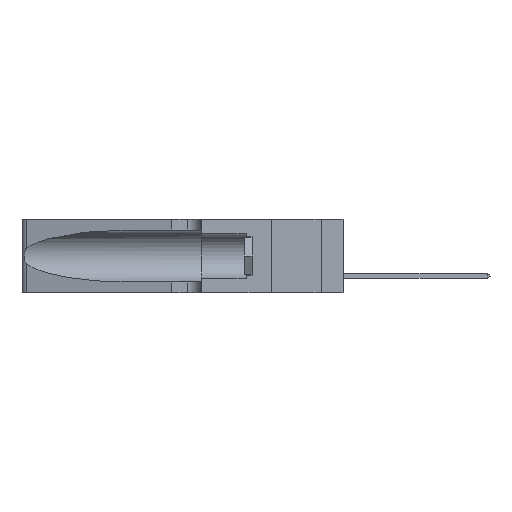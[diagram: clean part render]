
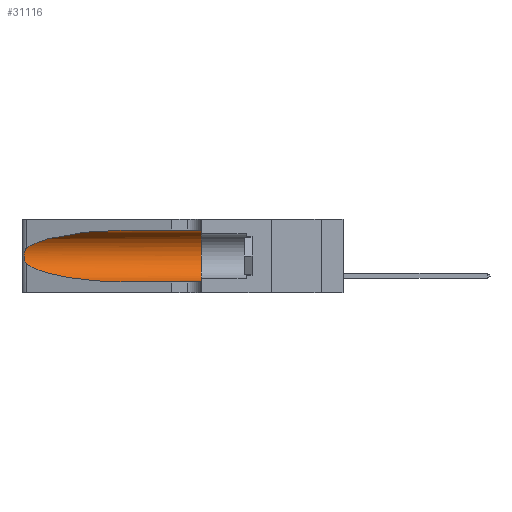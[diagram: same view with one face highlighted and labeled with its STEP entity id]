
A CAD part, left-side view. The second image highlights one B-rep face of the part: STEP entity #31116.
In plain terms, the highlighted cylindrical face has radius 3.308 mm (diameter 6.617 mm), a partial arc.
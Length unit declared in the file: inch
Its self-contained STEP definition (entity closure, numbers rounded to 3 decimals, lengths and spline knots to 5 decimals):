
#61 = CARTESIAN_POINT ( 'NONE',  ( 0.18966, 0.96281, 0.05475 ) ) ;
#992 = CARTESIAN_POINT ( 'NONE',  ( 0.1305, 1.61858, 0.185 ) ) ;
#1251 = CARTESIAN_POINT ( 'NONE',  ( 0.25787, 1.23484, 0.2124 ) ) ;
#2944 = CYLINDRICAL_SURFACE ( 'NONE', #26615, 0.13025 ) ;
#3702 = CARTESIAN_POINT ( 'NONE',  ( 0.25555, 1.22994, 0.2215 ) ) ;
#4380 = CARTESIAN_POINT ( 'NONE',  ( 0.26017, 1.23833, 0.17102 ) ) ;
#4405 = ORIENTED_EDGE ( 'NONE', *, *, #23463, .T. ) ;
#4521 = CARTESIAN_POINT ( 'NONE',  ( 0.1305, 0.72297, 0.31525 ) ) ;
#4695 = CARTESIAN_POINT ( 'NONE',  ( 0.1305, 1.61858, 0.05475 ) ) ;
#5345 = CARTESIAN_POINT ( 'NONE',  ( 0.25487, 1.22718, 0.14631 ) ) ;
#6553 = FACE_OUTER_BOUND ( 'NONE', #12564, .T. ) ;
#7436 = ORIENTED_EDGE ( 'NONE', *, *, #21412, .T. ) ;
#7670 = DIRECTION ( 'NONE',  ( 0., 1., 0. ) ) ;
#7796 = CARTESIAN_POINT ( 'NONE',  ( 0.1305, 0.72297, 0.05475 ) ) ;
#8293 = LINE ( 'NONE', #4695, #29169 ) ;
#8953 = B_SPLINE_CURVE_WITH_KNOTS ( 'NONE', 3,
 ( #18846, #3702, #11468, #1251, #16125, #27378, #21960, #14533, #4380, #16780, #16673, #17554, #22630, #30514 ),
 .UNSPECIFIED., .F., .F.,
 ( 4, 2, 2, 2, 2, 2, 4 ),
 ( 0., 0.00027, 0.00053, 0.00107, 0.0016, 0.00187, 0.00214 ),
 .UNSPECIFIED. ) ;
#9632 = VERTEX_POINT ( 'NONE', #17139 ) ;
#9759 = CARTESIAN_POINT ( 'NONE',  ( 0.1305, 0.72297, 0.31525 ) ) ;
#11220 = DIRECTION ( 'NONE',  ( 0., -1., 0. ) ) ;
#11468 = CARTESIAN_POINT ( 'NONE',  ( 0.25639, 1.23184, 0.21858 ) ) ;
#11655 = VERTEX_POINT ( 'NONE', #17692 ) ;
#11929 = CIRCLE ( 'NONE', #21301, 0.13025 ) ;
#12028 =( BOUNDED_CURVE ( )  B_SPLINE_CURVE ( 3, ( #9759, #17297, #27707, #24999 ),
 .UNSPECIFIED., .F., .F. ) 
 B_SPLINE_CURVE_WITH_KNOTS ( ( 4, 4 ),
 ( 1.5708, 2.84003 ),
 .UNSPECIFIED. ) 
 CURVE ( )  GEOMETRIC_REPRESENTATION_ITEM ( )  RATIONAL_B_SPLINE_CURVE ( ( 1., 0.87, 0.87, 1. ) ) 
 REPRESENTATION_ITEM ( '' )  );
#12421 = DIRECTION ( 'NONE',  ( 0., -1., 0. ) ) ;
#12564 = EDGE_LOOP ( 'NONE', ( #27322, #7436, #4405, #26340, #18048, #29147 ) ) ;
#13697 = VERTEX_POINT ( 'NONE', #16873 ) ;
#14533 = CARTESIAN_POINT ( 'NONE',  ( 0.26075, 1.23896, 0.178 ) ) ;
#14765 = EDGE_CURVE ( 'NONE', #15102, #9632, #19279, .T. ) ;
#15102 = VERTEX_POINT ( 'NONE', #4521 ) ;
#15492 =( BOUNDED_CURVE ( )  B_SPLINE_CURVE ( 3, ( #5345, #20778, #61, #7796 ),
 .UNSPECIFIED., .F., .F. ) 
 B_SPLINE_CURVE_WITH_KNOTS ( ( 4, 4 ),
 ( 3.44316, 4.71239 ),
 .UNSPECIFIED. ) 
 CURVE ( )  GEOMETRIC_REPRESENTATION_ITEM ( )  RATIONAL_B_SPLINE_CURVE ( ( 1., 0.87, 0.87, 1. ) ) 
 REPRESENTATION_ITEM ( '' )  );
#16125 = CARTESIAN_POINT ( 'NONE',  ( 0.25854, 1.2359, 0.20912 ) ) ;
#16673 = CARTESIAN_POINT ( 'NONE',  ( 0.25789, 1.23486, 0.15765 ) ) ;
#16780 = CARTESIAN_POINT ( 'NONE',  ( 0.25856, 1.23593, 0.16098 ) ) ;
#16837 = VECTOR ( 'NONE', #29332, 39.37008 ) ;
#16873 = CARTESIAN_POINT ( 'NONE',  ( 0.25487, 1.22718, 0.14631 ) ) ;
#17139 = CARTESIAN_POINT ( 'NONE',  ( 0.1305, 0.35, 0.31525 ) ) ;
#17297 = CARTESIAN_POINT ( 'NONE',  ( 0.18966, 0.96281, 0.31525 ) ) ;
#17554 = CARTESIAN_POINT ( 'NONE',  ( 0.25639, 1.23186, 0.15144 ) ) ;
#17692 = CARTESIAN_POINT ( 'NONE',  ( 0.1305, 0.72297, 0.05475 ) ) ;
#18048 = ORIENTED_EDGE ( 'NONE', *, *, #26138, .F. ) ;
#18659 = CARTESIAN_POINT ( 'NONE',  ( 0.25487, 1.22718, 0.22369 ) ) ;
#18846 = CARTESIAN_POINT ( 'NONE',  ( 0.25487, 1.22718, 0.22369 ) ) ;
#19176 = CARTESIAN_POINT ( 'NONE',  ( 0.1305, 0.35, 0.05475 ) ) ;
#19279 = LINE ( 'NONE', #23932, #16837 ) ;
#20454 = CARTESIAN_POINT ( 'NONE',  ( 0.1305, 0.35, 0.185 ) ) ;
#20710 = VERTEX_POINT ( 'NONE', #19176 ) ;
#20778 = CARTESIAN_POINT ( 'NONE',  ( 0.2373, 1.15595, 0.08982 ) ) ;
#21210 = VERTEX_POINT ( 'NONE', #18659 ) ;
#21301 = AXIS2_PLACEMENT_3D ( 'NONE', #20454, #7670, #25646 ) ;
#21412 = EDGE_CURVE ( 'NONE', #21210, #13697, #8953, .T. ) ;
#21578 = EDGE_CURVE ( 'NONE', #11655, #20710, #8293, .T. ) ;
#21960 = CARTESIAN_POINT ( 'NONE',  ( 0.26075, 1.23896, 0.19203 ) ) ;
#22630 = CARTESIAN_POINT ( 'NONE',  ( 0.25555, 1.22993, 0.14849 ) ) ;
#23463 = EDGE_CURVE ( 'NONE', #13697, #11655, #15492, .T. ) ;
#23932 = CARTESIAN_POINT ( 'NONE',  ( 0.1305, 1.61858, 0.31525 ) ) ;
#24999 = CARTESIAN_POINT ( 'NONE',  ( 0.25487, 1.22718, 0.22369 ) ) ;
#25646 = DIRECTION ( 'NONE',  ( 0., 0., 1. ) ) ;
#26138 = EDGE_CURVE ( 'NONE', #9632, #20710, #11929, .T. ) ;
#26340 = ORIENTED_EDGE ( 'NONE', *, *, #21578, .T. ) ;
#26372 = DIRECTION ( 'NONE',  ( 0., 0., -1. ) ) ;
#26615 = AXIS2_PLACEMENT_3D ( 'NONE', #992, #11220, #26372 ) ;
#27067 = EDGE_CURVE ( 'NONE', #15102, #21210, #12028, .T. ) ;
#27322 = ORIENTED_EDGE ( 'NONE', *, *, #27067, .T. ) ;
#27378 = CARTESIAN_POINT ( 'NONE',  ( 0.26018, 1.23835, 0.19895 ) ) ;
#27707 = CARTESIAN_POINT ( 'NONE',  ( 0.2373, 1.15595, 0.28018 ) ) ;
#29147 = ORIENTED_EDGE ( 'NONE', *, *, #14765, .F. ) ;
#29169 = VECTOR ( 'NONE', #12421, 39.37008 ) ;
#29332 = DIRECTION ( 'NONE',  ( 0., -1., 0. ) ) ;
#30514 = CARTESIAN_POINT ( 'NONE',  ( 0.25487, 1.22718, 0.14631 ) ) ;
#31116 = ADVANCED_FACE ( 'NONE', ( #6553 ), #2944, .F. ) ;
